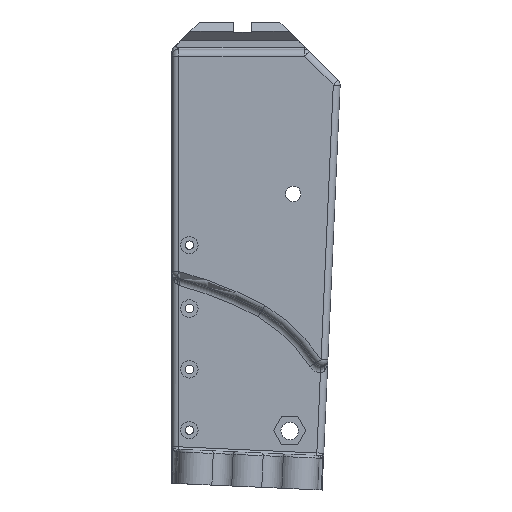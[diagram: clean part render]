
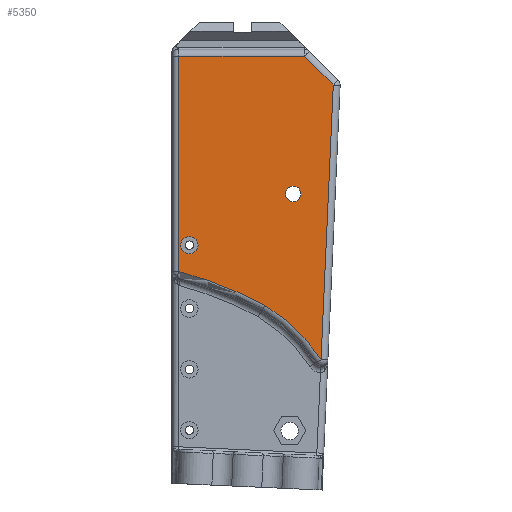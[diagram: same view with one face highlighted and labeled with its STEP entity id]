
A CAD part, left-side view. The second image highlights one B-rep face of the part: STEP entity #5350.
In plain terms, the highlighted planar face has unit normal (-1, 0, 0).
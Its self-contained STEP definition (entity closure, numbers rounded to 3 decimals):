
#82=FACE_BOUND('',#2138,.T.);
#83=FACE_BOUND('',#2139,.T.);
#323=LINE('',#32382,#638);
#324=LINE('',#32387,#639);
#325=LINE('',#32393,#640);
#527=LINE('',#34415,#842);
#638=VECTOR('',#6286,10.);
#639=VECTOR('',#6293,10.);
#640=VECTOR('',#6302,10.);
#842=VECTOR('',#7408,10.);
#1217=CIRCLE('',#5712,2.54);
#1218=CIRCLE('',#5713,2.54);
#1246=CIRCLE('',#5756,52.);
#1250=CIRCLE('',#5765,122.);
#1342=CIRCLE('',#5952,2.25);
#1769=FACE_OUTER_BOUND('',#2137,.T.);
#2137=EDGE_LOOP('',(#4900,#4901,#4902,#4903,#4904,#4905));
#2138=EDGE_LOOP('',(#4906));
#2139=EDGE_LOOP('',(#4907,#4908));
#2410=VERTEX_POINT('',#32365);
#2415=VERTEX_POINT('',#32381);
#2416=VERTEX_POINT('',#32385);
#2417=VERTEX_POINT('',#32391);
#2589=VERTEX_POINT('',#32953);
#2590=VERTEX_POINT('',#32954);
#2618=VERTEX_POINT('',#33032);
#2619=VERTEX_POINT('',#33034);
#2708=VERTEX_POINT('',#34407);
#2937=EDGE_CURVE('',#2410,#2415,#323,.T.);
#2940=EDGE_CURVE('',#2416,#2410,#324,.T.);
#2943=EDGE_CURVE('',#2417,#2416,#325,.T.);
#3205=EDGE_CURVE('',#2589,#2590,#1217,.T.);
#3207=EDGE_CURVE('',#2590,#2589,#1218,.T.);
#3242=EDGE_CURVE('',#2618,#2619,#1246,.T.);
#3249=EDGE_CURVE('',#2619,#2417,#1250,.T.);
#3440=EDGE_CURVE('',#2708,#2708,#1342,.T.);
#3444=EDGE_CURVE('',#2415,#2618,#527,.T.);
#4900=ORIENTED_EDGE('',*,*,#2943,.F.);
#4901=ORIENTED_EDGE('',*,*,#3249,.F.);
#4902=ORIENTED_EDGE('',*,*,#3242,.F.);
#4903=ORIENTED_EDGE('',*,*,#3444,.F.);
#4904=ORIENTED_EDGE('',*,*,#2937,.F.);
#4905=ORIENTED_EDGE('',*,*,#2940,.F.);
#4906=ORIENTED_EDGE('',*,*,#3440,.T.);
#4907=ORIENTED_EDGE('',*,*,#3205,.F.);
#4908=ORIENTED_EDGE('',*,*,#3207,.F.);
#5034=PLANE('',#5962);
#5350=ADVANCED_FACE('',(#1769,#82,#83),#5034,.F.);
#5712=AXIS2_PLACEMENT_3D('',#32955,#6857,#6858);
#5713=AXIS2_PLACEMENT_3D('',#32957,#6860,#6861);
#5756=AXIS2_PLACEMENT_3D('',#33035,#6952,#6953);
#5765=AXIS2_PLACEMENT_3D('',#33081,#6970,#6971);
#5952=AXIS2_PLACEMENT_3D('',#34408,#7399,#7400);
#5962=AXIS2_PLACEMENT_3D('',#34423,#7423,#7424);
#6286=DIRECTION('',(0.,-0.707,-0.707));
#6293=DIRECTION('',(0.,-1.,0.));
#6302=DIRECTION('',(0.,0.,1.));
#6857=DIRECTION('center_axis',(-1.,0.,0.));
#6858=DIRECTION('ref_axis',(0.,0.,-1.));
#6860=DIRECTION('center_axis',(-1.,0.,0.));
#6861=DIRECTION('ref_axis',(0.,0.,-1.));
#6952=DIRECTION('center_axis',(-1.,0.,0.));
#6953=DIRECTION('ref_axis',(0.,-0.742,0.67));
#6970=DIRECTION('center_axis',(-1.,0.,0.));
#6971=DIRECTION('ref_axis',(0.,-0.36,0.933));
#7399=DIRECTION('center_axis',(1.,0.,0.));
#7400=DIRECTION('ref_axis',(0.,0.,1.));
#7408=DIRECTION('',(0.,0.044,-0.999));
#7423=DIRECTION('center_axis',(1.,0.,0.));
#7424=DIRECTION('ref_axis',(0.,0.,-1.));
#32365=CARTESIAN_POINT('',(-30.1,-38.819,283.));
#32381=CARTESIAN_POINT('',(-30.1,-47.232,274.587));
#32382=CARTESIAN_POINT('',(-30.1,-48.759,273.06));
#32385=CARTESIAN_POINT('',(-30.1,-2.086,283.));
#32387=CARTESIAN_POINT('',(-30.1,-21.538,283.));
#32391=CARTESIAN_POINT('',(-30.1,-2.086,220.116));
#32393=CARTESIAN_POINT('',(-30.1,-2.086,121.679));
#32953=CARTESIAN_POINT('',(-30.1,-5.186,230.306));
#32954=CARTESIAN_POINT('',(-30.1,-5.186,225.226));
#32955=CARTESIAN_POINT('Origin',(-30.1,-5.186,227.766));
#32957=CARTESIAN_POINT('Origin',(-30.1,-5.186,227.766));
#33032=CARTESIAN_POINT('',(-30.1,-43.66,194.375));
#33034=CARTESIAN_POINT('',(-30.1,-27.248,210.212));
#33035=CARTESIAN_POINT('Origin',(-30.1,-0.224,165.785));
#33081=CARTESIAN_POINT('Origin',(-30.1,29.741,102.34));
#34407=CARTESIAN_POINT('',(-30.1,-35.522,240.525));
#34408=CARTESIAN_POINT('Origin',(-30.1,-35.522,242.775));
#34415=CARTESIAN_POINT('',(-30.1,-41.669,149.68));
#34423=CARTESIAN_POINT('Origin',(-30.1,-24.313,243.358));
